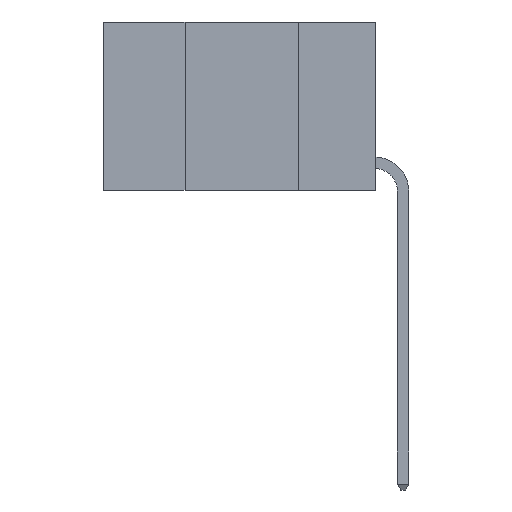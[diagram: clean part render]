
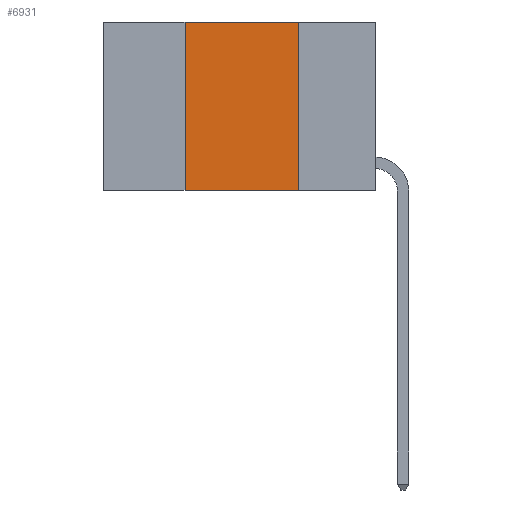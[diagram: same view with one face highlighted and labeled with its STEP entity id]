
A CAD part, left-side view. The second image highlights one B-rep face of the part: STEP entity #6931.
In plain terms, the highlighted planar face has unit normal (-1, 0, 0).
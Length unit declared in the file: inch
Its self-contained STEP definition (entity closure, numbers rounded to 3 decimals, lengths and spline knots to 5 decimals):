
#55 = VERTEX_POINT ( 'NONE', #9827 ) ;
#428 = DIRECTION ( 'NONE',  ( 0., 0., -1. ) ) ;
#456 = CARTESIAN_POINT ( 'NONE',  ( 0., 0.17, 0. ) ) ;
#973 = FACE_OUTER_BOUND ( 'NONE', #9720, .T. ) ;
#1083 = CARTESIAN_POINT ( 'NONE',  ( 0., 0.6, 0. ) ) ;
#1296 = DIRECTION ( 'NONE',  ( 1., 0., 0. ) ) ;
#1316 = CARTESIAN_POINT ( 'NONE',  ( 0., 0.17, -0.37 ) ) ;
#1384 = EDGE_CURVE ( 'NONE', #55, #2233, #10553, .T. ) ;
#1969 = LINE ( 'NONE', #6606, #11376 ) ;
#2233 = VERTEX_POINT ( 'NONE', #456 ) ;
#3461 = CARTESIAN_POINT ( 'NONE',  ( 0., 0.42, 0. ) ) ;
#3475 = EDGE_CURVE ( 'NONE', #2233, #6282, #1969, .T. ) ;
#3499 = DIRECTION ( 'NONE',  ( 0., 0., 1. ) ) ;
#4064 = EDGE_CURVE ( 'NONE', #9090, #55, #9694, .T. ) ;
#4084 = VECTOR ( 'NONE', #4320, 39.37008 ) ;
#4320 = DIRECTION ( 'NONE',  ( 0., -1., 0. ) ) ;
#6085 = AXIS2_PLACEMENT_3D ( 'NONE', #11012, #1296, #7504 ) ;
#6122 = VECTOR ( 'NONE', #6372, 39.37008 ) ;
#6180 = ORIENTED_EDGE ( 'NONE', *, *, #1384, .F. ) ;
#6282 = VERTEX_POINT ( 'NONE', #1316 ) ;
#6372 = DIRECTION ( 'NONE',  ( 0., -1., 0. ) ) ;
#6602 = PLANE ( 'NONE',  #6085 ) ;
#6606 = CARTESIAN_POINT ( 'NONE',  ( 0., 0.17, 0. ) ) ;
#6931 = ADVANCED_FACE ( 'NONE', ( #973 ), #6602, .F. ) ;
#7361 = VECTOR ( 'NONE', #3499, 39.37008 ) ;
#7504 = DIRECTION ( 'NONE',  ( 0., 0., -1. ) ) ;
#7866 = CARTESIAN_POINT ( 'NONE',  ( 0., 0.6, -0.37 ) ) ;
#7915 = CARTESIAN_POINT ( 'NONE',  ( 0., 0.42, -0.37 ) ) ;
#8573 = ORIENTED_EDGE ( 'NONE', *, *, #4064, .F. ) ;
#9090 = VERTEX_POINT ( 'NONE', #7915 ) ;
#9519 = ORIENTED_EDGE ( 'NONE', *, *, #10647, .T. ) ;
#9694 = LINE ( 'NONE', #3461, #7361 ) ;
#9720 = EDGE_LOOP ( 'NONE', ( #10902, #6180, #8573, #9519 ) ) ;
#9827 = CARTESIAN_POINT ( 'NONE',  ( 0., 0.42, 0. ) ) ;
#10553 = LINE ( 'NONE', #1083, #6122 ) ;
#10647 = EDGE_CURVE ( 'NONE', #9090, #6282, #11138, .T. ) ;
#10902 = ORIENTED_EDGE ( 'NONE', *, *, #3475, .F. ) ;
#11012 = CARTESIAN_POINT ( 'NONE',  ( 0., 0.6, 0. ) ) ;
#11138 = LINE ( 'NONE', #7866, #4084 ) ;
#11376 = VECTOR ( 'NONE', #428, 39.37008 ) ;
